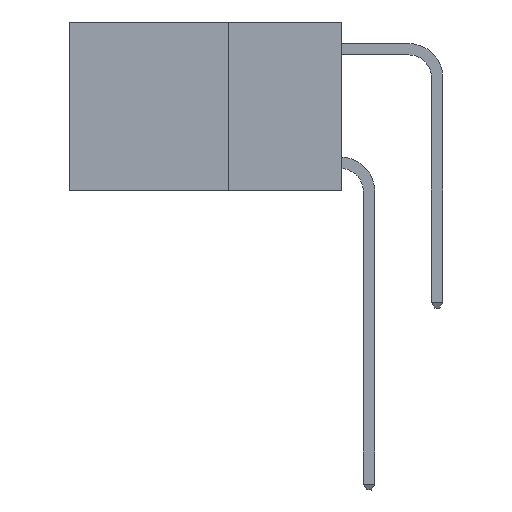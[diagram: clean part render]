
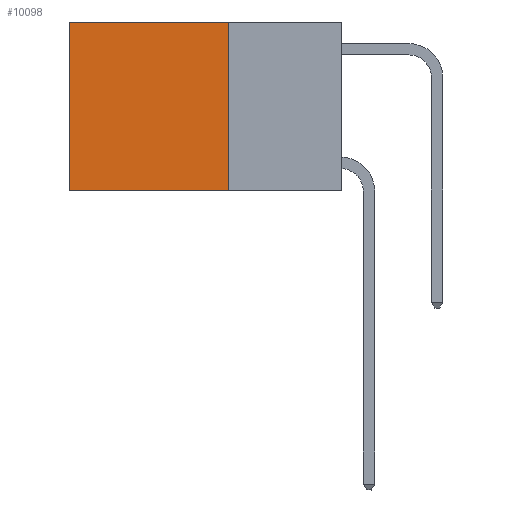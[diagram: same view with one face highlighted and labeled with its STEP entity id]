
A CAD part, left-side view. The second image highlights one B-rep face of the part: STEP entity #10098.
In plain terms, the highlighted planar face has unit normal (-1, 0, 0).
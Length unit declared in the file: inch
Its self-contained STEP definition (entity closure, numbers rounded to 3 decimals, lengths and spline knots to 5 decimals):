
#99 = VECTOR ( 'NONE', #5227, 39.37008 ) ;
#181 = VERTEX_POINT ( 'NONE', #856 ) ;
#856 = CARTESIAN_POINT ( 'NONE',  ( 0.2625, 0.25, -0.37 ) ) ;
#1679 = FACE_OUTER_BOUND ( 'NONE', #3551, .T. ) ;
#2677 = DIRECTION ( 'NONE',  ( 0., 0., -1. ) ) ;
#2705 = CARTESIAN_POINT ( 'NONE',  ( 0.2625, 0.25, -0.37 ) ) ;
#2982 = DIRECTION ( 'NONE',  ( 0., 0., -1. ) ) ;
#3033 = LINE ( 'NONE', #5027, #7627 ) ;
#3102 = EDGE_CURVE ( 'NONE', #10743, #4362, #3033, .T. ) ;
#3551 = EDGE_LOOP ( 'NONE', ( #10026, #5838, #4066, #10824 ) ) ;
#3991 = PLANE ( 'NONE',  #6488 ) ;
#4066 = ORIENTED_EDGE ( 'NONE', *, *, #9585, .F. ) ;
#4292 = VECTOR ( 'NONE', #2677, 39.37008 ) ;
#4362 = VERTEX_POINT ( 'NONE', #10674 ) ;
#4526 = LINE ( 'NONE', #2705, #99 ) ;
#5027 = CARTESIAN_POINT ( 'NONE',  ( 0.2625, 0.25, 0. ) ) ;
#5227 = DIRECTION ( 'NONE',  ( 0., 1., 0. ) ) ;
#5838 = ORIENTED_EDGE ( 'NONE', *, *, #9165, .F. ) ;
#6488 = AXIS2_PLACEMENT_3D ( 'NONE', #10804, #6500, #9155 ) ;
#6500 = DIRECTION ( 'NONE',  ( 1., 0., 0. ) ) ;
#6686 = CARTESIAN_POINT ( 'NONE',  ( 0.2625, 0.6, -0.37 ) ) ;
#6900 = LINE ( 'NONE', #8507, #4292 ) ;
#7627 = VECTOR ( 'NONE', #10962, 39.37008 ) ;
#7808 = VECTOR ( 'NONE', #2982, 39.37008 ) ;
#7847 = VERTEX_POINT ( 'NONE', #6686 ) ;
#8507 = CARTESIAN_POINT ( 'NONE',  ( 0.2625, 0.6, 0. ) ) ;
#8580 = CARTESIAN_POINT ( 'NONE',  ( 0.2625, 0.25, 0. ) ) ;
#8625 = LINE ( 'NONE', #9648, #7808 ) ;
#9155 = DIRECTION ( 'NONE',  ( 0., 0., -1. ) ) ;
#9165 = EDGE_CURVE ( 'NONE', #181, #7847, #4526, .T. ) ;
#9585 = EDGE_CURVE ( 'NONE', #10743, #181, #8625, .T. ) ;
#9648 = CARTESIAN_POINT ( 'NONE',  ( 0.2625, 0.25, 0. ) ) ;
#10026 = ORIENTED_EDGE ( 'NONE', *, *, #10702, .T. ) ;
#10098 = ADVANCED_FACE ( 'NONE', ( #1679 ), #3991, .F. ) ;
#10674 = CARTESIAN_POINT ( 'NONE',  ( 0.2625, 0.6, 0. ) ) ;
#10702 = EDGE_CURVE ( 'NONE', #4362, #7847, #6900, .T. ) ;
#10743 = VERTEX_POINT ( 'NONE', #8580 ) ;
#10804 = CARTESIAN_POINT ( 'NONE',  ( 0.2625, 0.25, 0. ) ) ;
#10824 = ORIENTED_EDGE ( 'NONE', *, *, #3102, .T. ) ;
#10962 = DIRECTION ( 'NONE',  ( 0., 1., 0. ) ) ;
